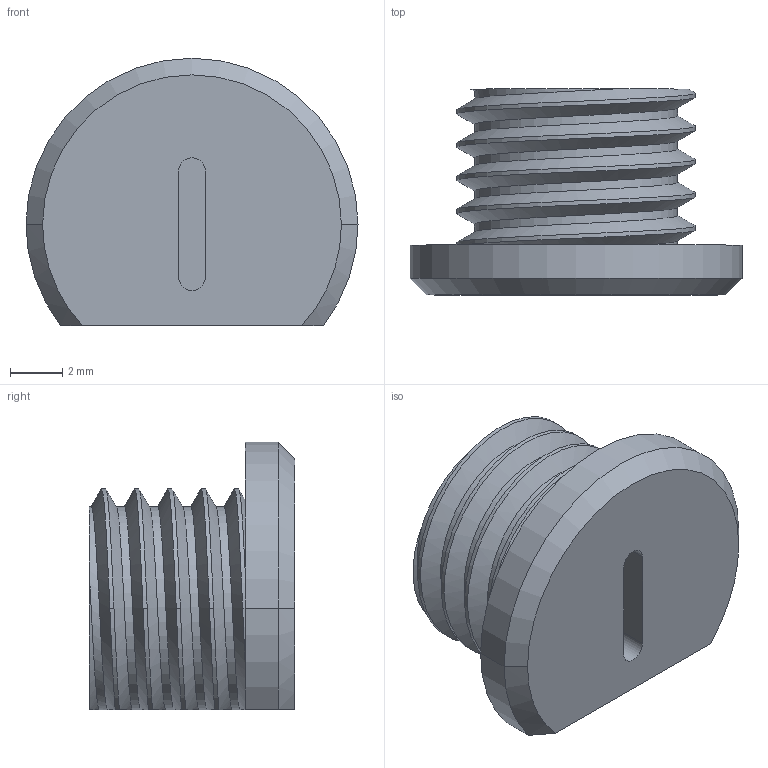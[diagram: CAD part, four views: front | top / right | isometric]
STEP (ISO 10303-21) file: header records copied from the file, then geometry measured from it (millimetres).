
FILE_DESCRIPTION (( 'STEP AP203' ), '1' );
FILE_NAME ('AF-WF-TC-PRT-002-STEP.STEP', '2020-07-22T00:08:52', ( '' ), ( '' ), 'SwSTEP 2.0', 'SolidWorks 2018', '' );
FILE_SCHEMA (( 'CONFIG_CONTROL_DESIGN' ));
Length unit declared in the file: inch
Products named in the file (1): AF-WF-TC-PRT-002-STEP
Bounding box: 12.7 x 7.87 x 10.23 mm (x, y, z)
Volume: 509 mm3; surface area: 566 mm2
Topology: 1 solids, 1 shells, 48 faces, 133 edges, 88 vertices
Faces by surface type: cylinder 20, bspline 18, plane 7, cone 3
Entity records: 5298 total; most frequent: CARTESIAN_POINT 4255, ORIENTED_EDGE 266, EDGE_CURVE 133, DIRECTION 131, VERTEX_POINT 88, EDGE_LOOP 49, FACE_OUTER_BOUND 48, ADVANCED_FACE 48
